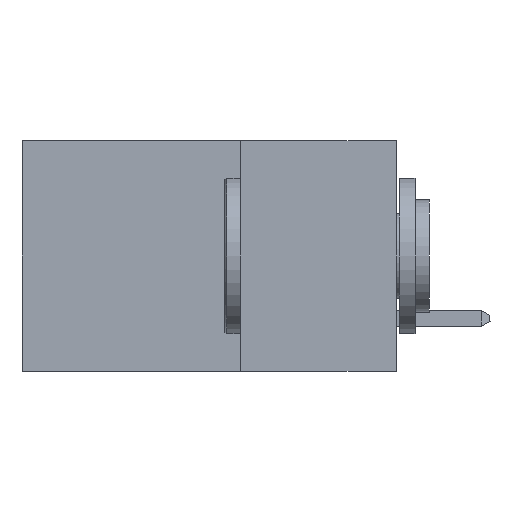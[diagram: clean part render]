
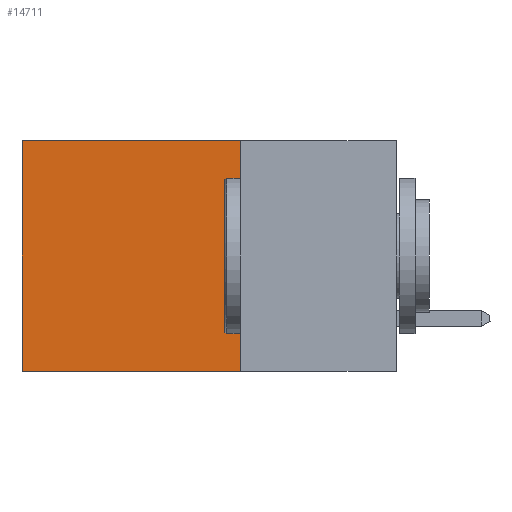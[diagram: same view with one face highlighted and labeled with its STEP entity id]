
A CAD part, left-side view. The second image highlights one B-rep face of the part: STEP entity #14711.
In plain terms, the highlighted planar face has unit normal (-1, 0, 0).
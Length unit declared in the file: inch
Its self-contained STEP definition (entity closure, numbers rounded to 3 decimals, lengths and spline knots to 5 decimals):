
#296 = CARTESIAN_POINT ( 'NONE',  ( 0.298, 0.6, 0. ) ) ;
#451 = ORIENTED_EDGE ( 'NONE', *, *, #7838, .T. ) ;
#1949 = CARTESIAN_POINT ( 'NONE',  ( 0.298, 0.6, -0.37 ) ) ;
#2044 = EDGE_CURVE ( 'NONE', #6007, #11975, #17284, .T. ) ;
#2427 = EDGE_CURVE ( 'NONE', #16298, #22601, #22441, .T. ) ;
#2482 = EDGE_LOOP ( 'NONE', ( #15692, #17091, #23075, #451 ) ) ;
#2524 = VECTOR ( 'NONE', #20074, 39.37008 ) ;
#2868 = DIRECTION ( 'NONE',  ( 1., 0., 0. ) ) ;
#4210 = CARTESIAN_POINT ( 'NONE',  ( 0.298, 0.25, 0. ) ) ;
#6007 = VERTEX_POINT ( 'NONE', #12948 ) ;
#6027 = LINE ( 'NONE', #15310, #10967 ) ;
#6110 = DIRECTION ( 'NONE',  ( 0., 1., 0. ) ) ;
#6882 = FACE_OUTER_BOUND ( 'NONE', #2482, .T. ) ;
#7838 = EDGE_CURVE ( 'NONE', #16298, #6007, #20760, .T. ) ;
#10279 = CARTESIAN_POINT ( 'NONE',  ( 0.298, 0.25, 0. ) ) ;
#10967 = VECTOR ( 'NONE', #6110, 39.37008 ) ;
#10980 = VECTOR ( 'NONE', #23174, 39.37008 ) ;
#11859 = CARTESIAN_POINT ( 'NONE',  ( 0.298, 0.25, -0.37 ) ) ;
#11975 = VERTEX_POINT ( 'NONE', #1949 ) ;
#12673 = VECTOR ( 'NONE', #18925, 39.37008 ) ;
#12948 = CARTESIAN_POINT ( 'NONE',  ( 0.298, 0.6, 0. ) ) ;
#13332 = AXIS2_PLACEMENT_3D ( 'NONE', #13946, #2868, #15774 ) ;
#13946 = CARTESIAN_POINT ( 'NONE',  ( 0.298, 0.25, 0. ) ) ;
#14564 = EDGE_CURVE ( 'NONE', #22601, #11975, #6027, .T. ) ;
#14711 = ADVANCED_FACE ( 'NONE', ( #6882 ), #23089, .F. ) ;
#15310 = CARTESIAN_POINT ( 'NONE',  ( 0.298, 0.25, -0.37 ) ) ;
#15692 = ORIENTED_EDGE ( 'NONE', *, *, #2044, .T. ) ;
#15774 = DIRECTION ( 'NONE',  ( 0., 0., -1. ) ) ;
#16298 = VERTEX_POINT ( 'NONE', #10279 ) ;
#17091 = ORIENTED_EDGE ( 'NONE', *, *, #14564, .F. ) ;
#17284 = LINE ( 'NONE', #296, #2524 ) ;
#18925 = DIRECTION ( 'NONE',  ( 0., 0., -1. ) ) ;
#20074 = DIRECTION ( 'NONE',  ( 0., 0., -1. ) ) ;
#20760 = LINE ( 'NONE', #21345, #10980 ) ;
#21345 = CARTESIAN_POINT ( 'NONE',  ( 0.298, 0.25, 0. ) ) ;
#22441 = LINE ( 'NONE', #4210, #12673 ) ;
#22601 = VERTEX_POINT ( 'NONE', #11859 ) ;
#23075 = ORIENTED_EDGE ( 'NONE', *, *, #2427, .F. ) ;
#23089 = PLANE ( 'NONE',  #13332 ) ;
#23174 = DIRECTION ( 'NONE',  ( 0., 1., 0. ) ) ;
